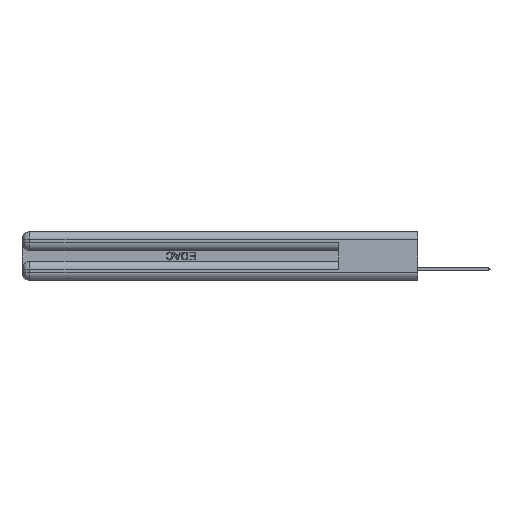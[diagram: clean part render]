
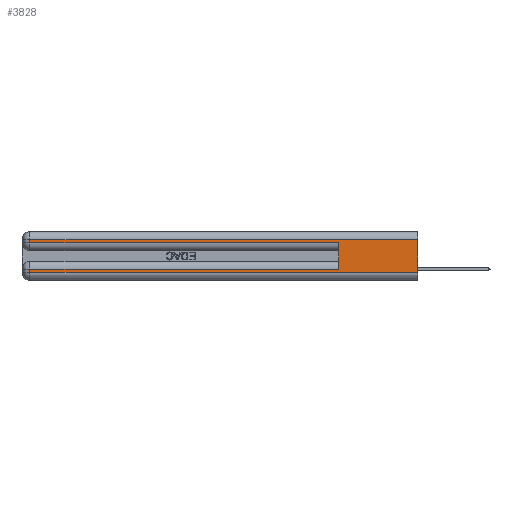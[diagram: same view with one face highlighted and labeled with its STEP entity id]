
A CAD part, left-side view. The second image highlights one B-rep face of the part: STEP entity #3828.
In plain terms, the highlighted planar face has unit normal (-1, 0, 0).
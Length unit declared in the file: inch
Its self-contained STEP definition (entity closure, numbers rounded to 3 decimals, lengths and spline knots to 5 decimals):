
#849 = CARTESIAN_POINT ( 'NONE',  ( 0., 2.94, 0.37 ) ) ;
#1288 = DIRECTION ( 'NONE',  ( 0., 1., 0. ) ) ;
#1705 = CARTESIAN_POINT ( 'NONE',  ( 0., 0., 0.285 ) ) ;
#2882 = VERTEX_POINT ( 'NONE', #3664 ) ;
#3558 = LINE ( 'NONE', #1705, #45759 ) ;
#3622 = EDGE_CURVE ( 'NONE', #7908, #9288, #28043, .T. ) ;
#3664 = CARTESIAN_POINT ( 'NONE',  ( 0., 2.94, 0.285 ) ) ;
#3828 = ADVANCED_FACE ( 'NONE', ( #20366 ), #6038, .F. ) ;
#5225 = CARTESIAN_POINT ( 'NONE',  ( 0., 0., 0.31 ) ) ;
#6038 = PLANE ( 'NONE',  #22650 ) ;
#6345 = VECTOR ( 'NONE', #18705, 39.37008 ) ;
#7908 = VERTEX_POINT ( 'NONE', #10490 ) ;
#8703 = ORIENTED_EDGE ( 'NONE', *, *, #25747, .T. ) ;
#9288 = VERTEX_POINT ( 'NONE', #32240 ) ;
#9498 = ORIENTED_EDGE ( 'NONE', *, *, #37601, .T. ) ;
#10124 = CARTESIAN_POINT ( 'NONE',  ( 0., 2.94, 0.085 ) ) ;
#10490 = CARTESIAN_POINT ( 'NONE',  ( 0., 0., 0.31 ) ) ;
#13421 = DIRECTION ( 'NONE',  ( 1., 0., 0. ) ) ;
#14092 = CARTESIAN_POINT ( 'NONE',  ( 0., 0., 0.06 ) ) ;
#16176 = EDGE_CURVE ( 'NONE', #47116, #18029, #38325, .T. ) ;
#16554 = VECTOR ( 'NONE', #42305, 39.37008 ) ;
#18029 = VERTEX_POINT ( 'NONE', #39280 ) ;
#18705 = DIRECTION ( 'NONE',  ( 0., 0., -1. ) ) ;
#19396 = ORIENTED_EDGE ( 'NONE', *, *, #16176, .T. ) ;
#20003 = CARTESIAN_POINT ( 'NONE',  ( 0., 0., 0.06 ) ) ;
#20008 = ORIENTED_EDGE ( 'NONE', *, *, #34907, .T. ) ;
#20189 = CARTESIAN_POINT ( 'NONE',  ( 0., 2.94, 0.37 ) ) ;
#20346 = DIRECTION ( 'NONE',  ( 0., 0., -1. ) ) ;
#20366 = FACE_OUTER_BOUND ( 'NONE', #29058, .T. ) ;
#20486 = EDGE_CURVE ( 'NONE', #18029, #31172, #29448, .T. ) ;
#20986 = CARTESIAN_POINT ( 'NONE',  ( 0., 0.6, 0.285 ) ) ;
#22650 = AXIS2_PLACEMENT_3D ( 'NONE', #35873, #13421, #43946 ) ;
#22877 = VERTEX_POINT ( 'NONE', #36302 ) ;
#22993 = ORIENTED_EDGE ( 'NONE', *, *, #3622, .T. ) ;
#23331 = CARTESIAN_POINT ( 'NONE',  ( 0., 0.6, 0.145 ) ) ;
#23991 = DIRECTION ( 'NONE',  ( 0., 0., -1. ) ) ;
#24811 = DIRECTION ( 'NONE',  ( 0., -1., 0. ) ) ;
#25702 = ORIENTED_EDGE ( 'NONE', *, *, #32651, .F. ) ;
#25747 = EDGE_CURVE ( 'NONE', #9288, #2882, #38353, .T. ) ;
#26379 = VERTEX_POINT ( 'NONE', #20986 ) ;
#27251 = LINE ( 'NONE', #27518, #29641 ) ;
#27518 = CARTESIAN_POINT ( 'NONE',  ( 0., 0., 0.085 ) ) ;
#28043 = LINE ( 'NONE', #5225, #32126 ) ;
#28803 = ORIENTED_EDGE ( 'NONE', *, *, #38231, .F. ) ;
#29058 = EDGE_LOOP ( 'NONE', ( #25702, #22993, #8703, #9498, #28803, #20008, #19396, #29622 ) ) ;
#29448 = LINE ( 'NONE', #20003, #16554 ) ;
#29622 = ORIENTED_EDGE ( 'NONE', *, *, #20486, .T. ) ;
#29641 = VECTOR ( 'NONE', #1288, 39.37008 ) ;
#31172 = VERTEX_POINT ( 'NONE', #14092 ) ;
#31272 = DIRECTION ( 'NONE',  ( 0., 1., 0. ) ) ;
#32126 = VECTOR ( 'NONE', #31272, 39.37008 ) ;
#32240 = CARTESIAN_POINT ( 'NONE',  ( 0., 2.94, 0.31 ) ) ;
#32651 = EDGE_CURVE ( 'NONE', #7908, #31172, #36279, .T. ) ;
#33450 = CARTESIAN_POINT ( 'NONE',  ( 0., 0., 0.37 ) ) ;
#34907 = EDGE_CURVE ( 'NONE', #22877, #47116, #27251, .T. ) ;
#35411 = VECTOR ( 'NONE', #20346, 39.37008 ) ;
#35873 = CARTESIAN_POINT ( 'NONE',  ( 0., 0., 0.37 ) ) ;
#36279 = LINE ( 'NONE', #33450, #6345 ) ;
#36302 = CARTESIAN_POINT ( 'NONE',  ( 0., 0.6, 0.085 ) ) ;
#37205 = VECTOR ( 'NONE', #23991, 39.37008 ) ;
#37601 = EDGE_CURVE ( 'NONE', #2882, #26379, #3558, .T. ) ;
#38231 = EDGE_CURVE ( 'NONE', #22877, #26379, #43747, .T. ) ;
#38325 = LINE ( 'NONE', #20189, #35411 ) ;
#38353 = LINE ( 'NONE', #849, #37205 ) ;
#38610 = DIRECTION ( 'NONE',  ( 0., 0., 1. ) ) ;
#39280 = CARTESIAN_POINT ( 'NONE',  ( 0., 2.94, 0.06 ) ) ;
#42305 = DIRECTION ( 'NONE',  ( 0., -1., 0. ) ) ;
#43747 = LINE ( 'NONE', #23331, #47226 ) ;
#43946 = DIRECTION ( 'NONE',  ( 0., 0., -1. ) ) ;
#45759 = VECTOR ( 'NONE', #24811, 39.37008 ) ;
#47116 = VERTEX_POINT ( 'NONE', #10124 ) ;
#47226 = VECTOR ( 'NONE', #38610, 39.37008 ) ;
